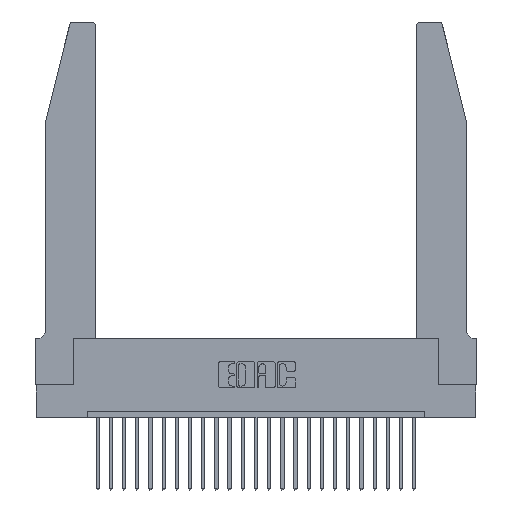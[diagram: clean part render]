
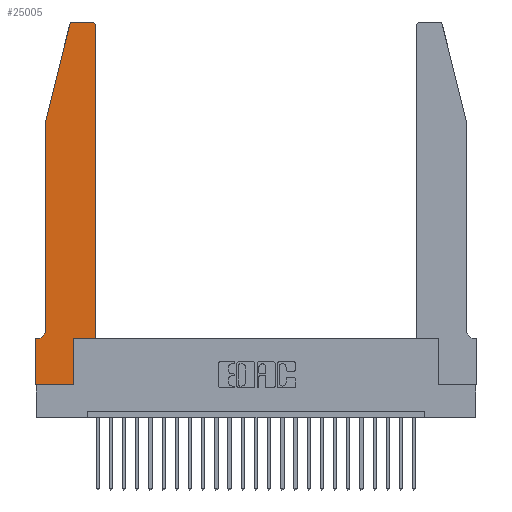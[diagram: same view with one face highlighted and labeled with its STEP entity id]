
A CAD part, top view. The second image highlights one B-rep face of the part: STEP entity #25005.
In plain terms, the highlighted planar face has unit normal (0, 0, 1).
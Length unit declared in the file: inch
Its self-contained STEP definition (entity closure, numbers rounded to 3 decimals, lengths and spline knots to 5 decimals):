
#789 = ORIENTED_EDGE ( 'NONE', *, *, #10020, .T. ) ;
#1004 = LINE ( 'NONE', #23773, #8466 ) ;
#1514 = VERTEX_POINT ( 'NONE', #8018 ) ;
#2000 = VERTEX_POINT ( 'NONE', #21559 ) ;
#2377 = EDGE_CURVE ( 'NONE', #7898, #19595, #23138, .T. ) ;
#2675 = EDGE_CURVE ( 'NONE', #12545, #25140, #12166, .T. ) ;
#3104 = EDGE_CURVE ( 'NONE', #22453, #12545, #7781, .T. ) ;
#3199 = CARTESIAN_POINT ( 'NONE',  ( 0.4505, 2.72, 0.37 ) ) ;
#3288 = DIRECTION ( 'NONE',  ( 0., 0., 1. ) ) ;
#3435 = ORIENTED_EDGE ( 'NONE', *, *, #25715, .T. ) ;
#3452 = VECTOR ( 'NONE', #20107, 39.37008 ) ;
#3463 = DIRECTION ( 'NONE',  ( -1., 0., 0. ) ) ;
#3520 = CARTESIAN_POINT ( 'NONE',  ( 0.0055, 0.35, 0.37 ) ) ;
#3699 = EDGE_CURVE ( 'NONE', #2000, #8367, #22436, .T. ) ;
#4158 = DIRECTION ( 'NONE',  ( 0., 0., -1. ) ) ;
#4588 = DIRECTION ( 'NONE',  ( -1., 0., 0. ) ) ;
#4658 = AXIS2_PLACEMENT_3D ( 'NONE', #16084, #4158, #10074 ) ;
#5164 = VERTEX_POINT ( 'NONE', #3199 ) ;
#5194 = EDGE_CURVE ( 'NONE', #5164, #7466, #22969, .T. ) ;
#5298 = ORIENTED_EDGE ( 'NONE', *, *, #2675, .T. ) ;
#5493 = AXIS2_PLACEMENT_3D ( 'NONE', #7992, #23564, #11939 ) ;
#6056 = EDGE_CURVE ( 'NONE', #25140, #1514, #14471, .T. ) ;
#7466 = VERTEX_POINT ( 'NONE', #24885 ) ;
#7554 = VECTOR ( 'NONE', #4588, 39.37008 ) ;
#7781 = LINE ( 'NONE', #25651, #21232 ) ;
#7898 = VERTEX_POINT ( 'NONE', #3520 ) ;
#7992 = CARTESIAN_POINT ( 'NONE',  ( 0., 0.35, 0.37 ) ) ;
#8018 = CARTESIAN_POINT ( 'NONE',  ( 0.4505, 0.35, 0.37 ) ) ;
#8080 = VECTOR ( 'NONE', #12572, 39.37008 ) ;
#8179 = CARTESIAN_POINT ( 'NONE',  ( 0.4505, 0.35, 0.37 ) ) ;
#8367 = VERTEX_POINT ( 'NONE', #18720 ) ;
#8466 = VECTOR ( 'NONE', #25855, 39.37008 ) ;
#9698 = VERTEX_POINT ( 'NONE', #16831 ) ;
#9801 = CARTESIAN_POINT ( 'NONE',  ( 0.0755, 2., 0.37 ) ) ;
#10020 = EDGE_CURVE ( 'NONE', #19595, #22453, #1004, .T. ) ;
#10074 = DIRECTION ( 'NONE',  ( -1., 0., 0. ) ) ;
#10165 = EDGE_LOOP ( 'NONE', ( #12035, #18775, #19378, #11377, #3435, #24356, #789, #12555, #5298, #20066, #11755, #10182 ) ) ;
#10182 = ORIENTED_EDGE ( 'NONE', *, *, #5194, .T. ) ;
#10301 = EDGE_CURVE ( 'NONE', #7466, #2000, #21937, .T. ) ;
#10801 = AXIS2_PLACEMENT_3D ( 'NONE', #17385, #3288, #19234 ) ;
#11377 = ORIENTED_EDGE ( 'NONE', *, *, #11772, .T. ) ;
#11755 = ORIENTED_EDGE ( 'NONE', *, *, #19080, .T. ) ;
#11772 = EDGE_CURVE ( 'NONE', #22940, #9698, #23696, .T. ) ;
#11818 = DIRECTION ( 'NONE',  ( -0.239, -0.971, 0. ) ) ;
#11939 = DIRECTION ( 'NONE',  ( 1., 0., 0. ) ) ;
#12035 = ORIENTED_EDGE ( 'NONE', *, *, #10301, .T. ) ;
#12166 = LINE ( 'NONE', #23343, #3452 ) ;
#12545 = VERTEX_POINT ( 'NONE', #13671 ) ;
#12555 = ORIENTED_EDGE ( 'NONE', *, *, #3104, .T. ) ;
#12572 = DIRECTION ( 'NONE',  ( 0., -1., 0. ) ) ;
#12657 = CARTESIAN_POINT ( 'NONE',  ( 0.0755, 2., 0.37 ) ) ;
#12909 = VECTOR ( 'NONE', #20071, 39.37008 ) ;
#13140 = CARTESIAN_POINT ( 'NONE',  ( 0.0755, 2., 0.37 ) ) ;
#13535 = CIRCLE ( 'NONE', #4658, 0.07 ) ;
#13667 = DIRECTION ( 'NONE',  ( 1., 0., 0. ) ) ;
#13671 = CARTESIAN_POINT ( 'NONE',  ( 0.2865, 0., 0.37 ) ) ;
#13722 = VECTOR ( 'NONE', #3463, 39.37008 ) ;
#13844 = PLANE ( 'NONE',  #5493 ) ;
#13994 = CARTESIAN_POINT ( 'NONE',  ( 0., 0.35, 0.37 ) ) ;
#14471 = LINE ( 'NONE', #8179, #12909 ) ;
#15624 = VECTOR ( 'NONE', #11818, 39.37008 ) ;
#15935 = CARTESIAN_POINT ( 'NONE',  ( 0.4505, 0.35, 0.37 ) ) ;
#16084 = CARTESIAN_POINT ( 'NONE',  ( 0.0055, 0.42, 0.37 ) ) ;
#16544 = CARTESIAN_POINT ( 'NONE',  ( 0.2605, 2.75, 0.37 ) ) ;
#16831 = CARTESIAN_POINT ( 'NONE',  ( 0.0755, 0.42, 0.37 ) ) ;
#17120 = DIRECTION ( 'NONE',  ( 1., 0., 0. ) ) ;
#17385 = CARTESIAN_POINT ( 'NONE',  ( 0.4205, 2.72, 0.37 ) ) ;
#18304 = CARTESIAN_POINT ( 'NONE',  ( 0.2865, 0.35, 0.37 ) ) ;
#18720 = CARTESIAN_POINT ( 'NONE',  ( 0.25487, 2.72718, 0.37 ) ) ;
#18775 = ORIENTED_EDGE ( 'NONE', *, *, #3699, .T. ) ;
#19080 = EDGE_CURVE ( 'NONE', #1514, #5164, #19104, .T. ) ;
#19104 = LINE ( 'NONE', #15935, #21298 ) ;
#19234 = DIRECTION ( 'NONE',  ( 1., 0., 0. ) ) ;
#19378 = ORIENTED_EDGE ( 'NONE', *, *, #19511, .T. ) ;
#19511 = EDGE_CURVE ( 'NONE', #8367, #22940, #20656, .T. ) ;
#19595 = VERTEX_POINT ( 'NONE', #13994 ) ;
#20066 = ORIENTED_EDGE ( 'NONE', *, *, #6056, .T. ) ;
#20071 = DIRECTION ( 'NONE',  ( 1., 0., 0. ) ) ;
#20107 = DIRECTION ( 'NONE',  ( 0., 1., 0. ) ) ;
#20656 = LINE ( 'NONE', #9801, #15624 ) ;
#21232 = VECTOR ( 'NONE', #13667, 39.37008 ) ;
#21298 = VECTOR ( 'NONE', #23975, 39.37008 ) ;
#21559 = CARTESIAN_POINT ( 'NONE',  ( 0.284, 2.75, 0.37 ) ) ;
#21937 = LINE ( 'NONE', #16544, #7554 ) ;
#22042 = FACE_OUTER_BOUND ( 'NONE', #10165, .T. ) ;
#22436 = CIRCLE ( 'NONE', #24962, 0.03 ) ;
#22453 = VERTEX_POINT ( 'NONE', #23510 ) ;
#22529 = DIRECTION ( 'NONE',  ( 0., 0., 1. ) ) ;
#22716 = CARTESIAN_POINT ( 'NONE',  ( 0.284, 2.72, 0.37 ) ) ;
#22940 = VERTEX_POINT ( 'NONE', #13140 ) ;
#22969 = CIRCLE ( 'NONE', #10801, 0.03 ) ;
#23138 = LINE ( 'NONE', #25503, #13722 ) ;
#23343 = CARTESIAN_POINT ( 'NONE',  ( 0.2865, 0.35, 0.37 ) ) ;
#23510 = CARTESIAN_POINT ( 'NONE',  ( 0., 0., 0.37 ) ) ;
#23564 = DIRECTION ( 'NONE',  ( 0., 0., 1. ) ) ;
#23696 = LINE ( 'NONE', #12657, #8080 ) ;
#23773 = CARTESIAN_POINT ( 'NONE',  ( 0., 0., 0.37 ) ) ;
#23975 = DIRECTION ( 'NONE',  ( 0., 1., 0. ) ) ;
#24356 = ORIENTED_EDGE ( 'NONE', *, *, #2377, .T. ) ;
#24885 = CARTESIAN_POINT ( 'NONE',  ( 0.4205, 2.75, 0.37 ) ) ;
#24962 = AXIS2_PLACEMENT_3D ( 'NONE', #22716, #22529, #17120 ) ;
#25005 = ADVANCED_FACE ( 'NONE', ( #22042 ), #13844, .T. ) ;
#25140 = VERTEX_POINT ( 'NONE', #18304 ) ;
#25503 = CARTESIAN_POINT ( 'NONE',  ( 0.0755, 0.35, 0.37 ) ) ;
#25651 = CARTESIAN_POINT ( 'NONE',  ( 0., 0., 0.37 ) ) ;
#25715 = EDGE_CURVE ( 'NONE', #9698, #7898, #13535, .T. ) ;
#25855 = DIRECTION ( 'NONE',  ( 0., -1., 0. ) ) ;
